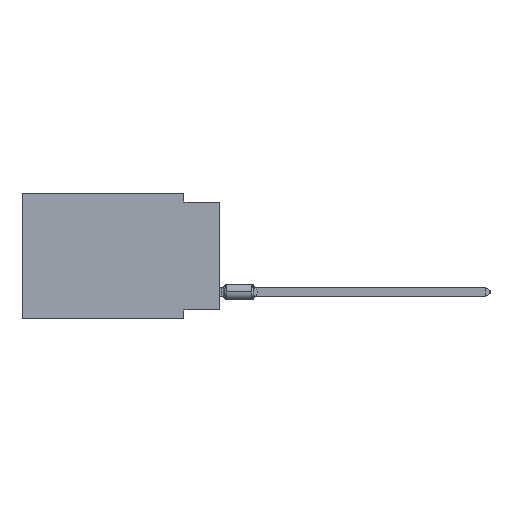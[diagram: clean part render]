
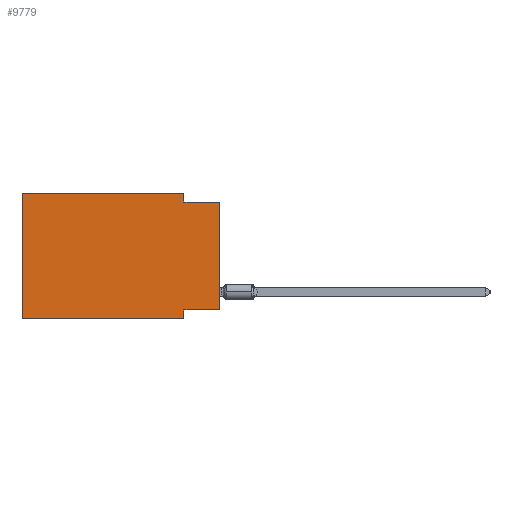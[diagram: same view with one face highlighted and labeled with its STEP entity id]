
A CAD part, left-side view. The second image highlights one B-rep face of the part: STEP entity #9779.
In plain terms, the highlighted planar face has unit normal (-1, 0, 0).
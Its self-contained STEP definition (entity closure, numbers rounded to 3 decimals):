
#339 = VERTEX_POINT ( 'NONE', #56333 ) ;
#578 = CARTESIAN_POINT ( 'NONE',  ( 0., 2.54, -8.255 ) ) ;
#1510 = FACE_OUTER_BOUND ( 'NONE', #21887, .T. ) ;
#2401 = PLANE ( 'NONE',  #40186 ) ;
#2907 = CARTESIAN_POINT ( 'NONE',  ( 0., 0., -0.635 ) ) ;
#3386 = VERTEX_POINT ( 'NONE', #29055 ) ;
#3409 = EDGE_CURVE ( 'NONE', #57201, #54750, #57398, .T. ) ;
#5025 = ORIENTED_EDGE ( 'NONE', *, *, #31382, .F. ) ;
#5240 = CARTESIAN_POINT ( 'NONE',  ( 0., 0., -8.255 ) ) ;
#5853 = CARTESIAN_POINT ( 'NONE',  ( 0., 13.97, 0. ) ) ;
#6510 = EDGE_CURVE ( 'NONE', #37184, #16236, #37887, .T. ) ;
#7446 = LINE ( 'NONE', #43695, #38155 ) ;
#9779 = ADVANCED_FACE ( 'NONE', ( #1510 ), #2401, .F. ) ;
#10187 = VECTOR ( 'NONE', #43962, 1000. ) ;
#10941 = LINE ( 'NONE', #48097, #14154 ) ;
#11238 = DIRECTION ( 'NONE',  ( 0., 0., -1. ) ) ;
#14154 = VECTOR ( 'NONE', #48982, 1000. ) ;
#14177 = EDGE_CURVE ( 'NONE', #339, #36803, #10941, .T. ) ;
#14648 = ORIENTED_EDGE ( 'NONE', *, *, #59327, .F. ) ;
#15798 = ORIENTED_EDGE ( 'NONE', *, *, #6510, .F. ) ;
#16236 = VERTEX_POINT ( 'NONE', #578 ) ;
#17511 = CARTESIAN_POINT ( 'NONE',  ( 0., 13.97, 0. ) ) ;
#18495 = VERTEX_POINT ( 'NONE', #53661 ) ;
#20072 = CARTESIAN_POINT ( 'NONE',  ( 0., 13.97, 0. ) ) ;
#20958 = DIRECTION ( 'NONE',  ( 1., 0., 0. ) ) ;
#21887 = EDGE_LOOP ( 'NONE', ( #29713, #14648, #42833, #33431, #51235, #25798, #5025, #15798 ) ) ;
#25030 = CARTESIAN_POINT ( 'NONE',  ( 0., 2.54, -8.89 ) ) ;
#25798 = ORIENTED_EDGE ( 'NONE', *, *, #3409, .T. ) ;
#29055 = CARTESIAN_POINT ( 'NONE',  ( 0., 13.97, 0. ) ) ;
#29363 = CARTESIAN_POINT ( 'NONE',  ( 0., 13.97, -8.89 ) ) ;
#29713 = ORIENTED_EDGE ( 'NONE', *, *, #59098, .T. ) ;
#31382 = EDGE_CURVE ( 'NONE', #16236, #54750, #7446, .T. ) ;
#32145 = VECTOR ( 'NONE', #49197, 1000. ) ;
#33233 = VECTOR ( 'NONE', #60162, 1000. ) ;
#33431 = ORIENTED_EDGE ( 'NONE', *, *, #41914, .F. ) ;
#35039 = LINE ( 'NONE', #5853, #45734 ) ;
#36803 = VERTEX_POINT ( 'NONE', #56165 ) ;
#37184 = VERTEX_POINT ( 'NONE', #5240 ) ;
#37887 = LINE ( 'NONE', #56493, #33233 ) ;
#38155 = VECTOR ( 'NONE', #48861, 1000. ) ;
#38857 = CARTESIAN_POINT ( 'NONE',  ( 0., 0., 0. ) ) ;
#39162 = DIRECTION ( 'NONE',  ( 0., 0., 1. ) ) ;
#39884 = VECTOR ( 'NONE', #39162, 1000. ) ;
#40186 = AXIS2_PLACEMENT_3D ( 'NONE', #20072, #20958, #11238 ) ;
#41914 = EDGE_CURVE ( 'NONE', #3386, #339, #50401, .T. ) ;
#42680 = EDGE_CURVE ( 'NONE', #57201, #3386, #35039, .T. ) ;
#42833 = ORIENTED_EDGE ( 'NONE', *, *, #14177, .F. ) ;
#42986 = DIRECTION ( 'NONE',  ( 0., 0., 1. ) ) ;
#43695 = CARTESIAN_POINT ( 'NONE',  ( 0., 2.54, -8.89 ) ) ;
#43962 = DIRECTION ( 'NONE',  ( 0., -1., 0. ) ) ;
#45734 = VECTOR ( 'NONE', #42986, 1000. ) ;
#46633 = VECTOR ( 'NONE', #50106, 1000. ) ;
#47360 = CARTESIAN_POINT ( 'NONE',  ( 0., 13.97, -8.89 ) ) ;
#48097 = CARTESIAN_POINT ( 'NONE',  ( 0., 2.54, 0. ) ) ;
#48861 = DIRECTION ( 'NONE',  ( 0., 0., -1. ) ) ;
#48982 = DIRECTION ( 'NONE',  ( 0., 0., -1. ) ) ;
#49197 = DIRECTION ( 'NONE',  ( 0., -1., 0. ) ) ;
#50106 = DIRECTION ( 'NONE',  ( 0., -1., 0. ) ) ;
#50401 = LINE ( 'NONE', #17511, #46633 ) ;
#51235 = ORIENTED_EDGE ( 'NONE', *, *, #42680, .F. ) ;
#53661 = CARTESIAN_POINT ( 'NONE',  ( 0., 0., -0.635 ) ) ;
#53774 = LINE ( 'NONE', #38857, #39884 ) ;
#54372 = LINE ( 'NONE', #2907, #32145 ) ;
#54750 = VERTEX_POINT ( 'NONE', #25030 ) ;
#56165 = CARTESIAN_POINT ( 'NONE',  ( 0., 2.54, -0.635 ) ) ;
#56333 = CARTESIAN_POINT ( 'NONE',  ( 0., 2.54, 0. ) ) ;
#56493 = CARTESIAN_POINT ( 'NONE',  ( 0., 0., -8.255 ) ) ;
#57201 = VERTEX_POINT ( 'NONE', #47360 ) ;
#57398 = LINE ( 'NONE', #29363, #10187 ) ;
#59098 = EDGE_CURVE ( 'NONE', #37184, #18495, #53774, .T. ) ;
#59327 = EDGE_CURVE ( 'NONE', #36803, #18495, #54372, .T. ) ;
#60162 = DIRECTION ( 'NONE',  ( 0., 1., 0. ) ) ;
